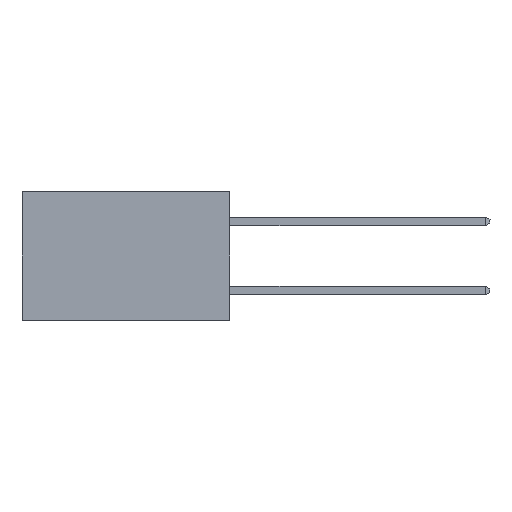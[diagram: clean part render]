
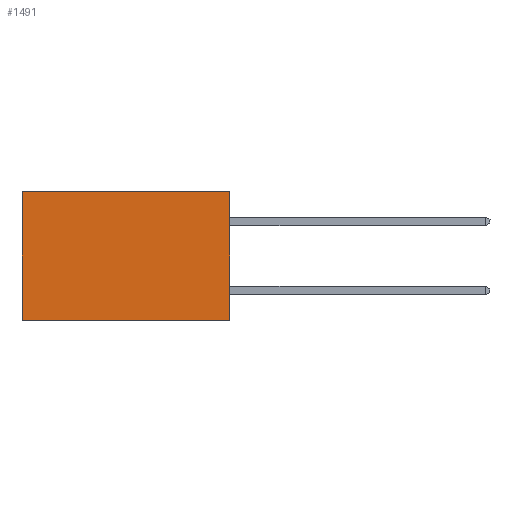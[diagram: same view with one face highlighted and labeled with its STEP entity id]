
A CAD part, left-side view. The second image highlights one B-rep face of the part: STEP entity #1491.
In plain terms, the highlighted planar face has unit normal (-1, 0, 0).
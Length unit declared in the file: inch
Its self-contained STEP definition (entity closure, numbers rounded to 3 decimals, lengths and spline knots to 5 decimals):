
#9 = LINE ( 'NONE', #5034, #2470 ) ;
#683 = CARTESIAN_POINT ( 'NONE',  ( 0.2615, 0., 0. ) ) ;
#1011 = CARTESIAN_POINT ( 'NONE',  ( 0.2615, 0., -0.37 ) ) ;
#1047 = EDGE_CURVE ( 'NONE', #7483, #3937, #1889, .T. ) ;
#1104 = DIRECTION ( 'NONE',  ( 1., 0., 0. ) ) ;
#1248 = LINE ( 'NONE', #6239, #4466 ) ;
#1491 = ADVANCED_FACE ( 'NONE', ( #2826 ), #4748, .F. ) ;
#1582 = CARTESIAN_POINT ( 'NONE',  ( 0.2615, 0.6, -0.37 ) ) ;
#1672 = CARTESIAN_POINT ( 'NONE',  ( 0.2615, 0., -0.37 ) ) ;
#1877 = CARTESIAN_POINT ( 'NONE',  ( 0.2615, 0., 0. ) ) ;
#1889 = LINE ( 'NONE', #683, #3203 ) ;
#2337 = EDGE_CURVE ( 'NONE', #7483, #2749, #1248, .T. ) ;
#2358 = DIRECTION ( 'NONE',  ( 0., 0., -1. ) ) ;
#2470 = VECTOR ( 'NONE', #7508, 39.37008 ) ;
#2749 = VERTEX_POINT ( 'NONE', #1672 ) ;
#2826 = FACE_OUTER_BOUND ( 'NONE', #5964, .T. ) ;
#2918 = DIRECTION ( 'NONE',  ( 0., 0., -1. ) ) ;
#3203 = VECTOR ( 'NONE', #6314, 39.37008 ) ;
#3261 = ORIENTED_EDGE ( 'NONE', *, *, #2337, .F. ) ;
#3937 = VERTEX_POINT ( 'NONE', #7085 ) ;
#4466 = VECTOR ( 'NONE', #2358, 39.37008 ) ;
#4748 = PLANE ( 'NONE',  #4979 ) ;
#4802 = ORIENTED_EDGE ( 'NONE', *, *, #1047, .T. ) ;
#4979 = AXIS2_PLACEMENT_3D ( 'NONE', #1011, #1104, #2918 ) ;
#5034 = CARTESIAN_POINT ( 'NONE',  ( 0.2615, 0., -0.37 ) ) ;
#5121 = CARTESIAN_POINT ( 'NONE',  ( 0.2615, 0.6, -0.37 ) ) ;
#5226 = VECTOR ( 'NONE', #5884, 39.37008 ) ;
#5884 = DIRECTION ( 'NONE',  ( 0., 0., -1. ) ) ;
#5964 = EDGE_LOOP ( 'NONE', ( #7608, #7013, #3261, #4802 ) ) ;
#6239 = CARTESIAN_POINT ( 'NONE',  ( 0.2615, 0., -0.37 ) ) ;
#6314 = DIRECTION ( 'NONE',  ( 0., 1., 0. ) ) ;
#6889 = EDGE_CURVE ( 'NONE', #3937, #7680, #7715, .T. ) ;
#7013 = ORIENTED_EDGE ( 'NONE', *, *, #7258, .F. ) ;
#7085 = CARTESIAN_POINT ( 'NONE',  ( 0.2615, 0.6, 0. ) ) ;
#7258 = EDGE_CURVE ( 'NONE', #2749, #7680, #9, .T. ) ;
#7483 = VERTEX_POINT ( 'NONE', #1877 ) ;
#7508 = DIRECTION ( 'NONE',  ( 0., 1., 0. ) ) ;
#7608 = ORIENTED_EDGE ( 'NONE', *, *, #6889, .T. ) ;
#7680 = VERTEX_POINT ( 'NONE', #1582 ) ;
#7715 = LINE ( 'NONE', #5121, #5226 ) ;
